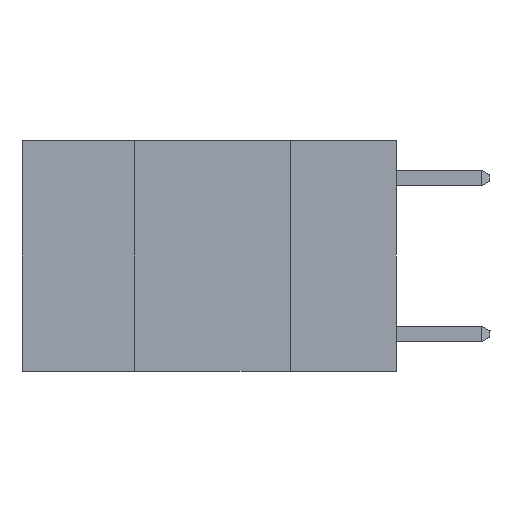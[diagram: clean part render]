
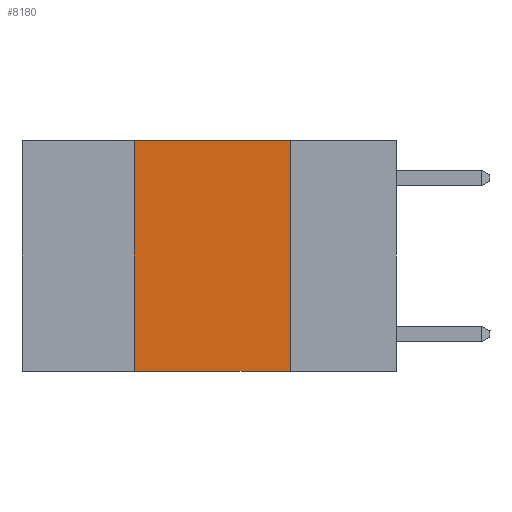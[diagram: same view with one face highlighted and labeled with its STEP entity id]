
A CAD part, left-side view. The second image highlights one B-rep face of the part: STEP entity #8180.
In plain terms, the highlighted planar face has unit normal (-1, 0, 0).
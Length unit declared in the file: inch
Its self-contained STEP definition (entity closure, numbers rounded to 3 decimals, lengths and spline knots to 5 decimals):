
#717 = CARTESIAN_POINT ( 'NONE',  ( 0., 0.42, 0. ) ) ;
#857 = LINE ( 'NONE', #12885, #6156 ) ;
#988 = CARTESIAN_POINT ( 'NONE',  ( 0., 0.6, -0.37 ) ) ;
#1146 = PLANE ( 'NONE',  #7755 ) ;
#1950 = LINE ( 'NONE', #988, #4448 ) ;
#2814 = CARTESIAN_POINT ( 'NONE',  ( 0., 0.17, 0. ) ) ;
#3198 = VERTEX_POINT ( 'NONE', #9468 ) ;
#3977 = EDGE_LOOP ( 'NONE', ( #6904, #7566, #7643, #7690 ) ) ;
#3981 = VERTEX_POINT ( 'NONE', #2814 ) ;
#4067 = CARTESIAN_POINT ( 'NONE',  ( 0., 0.6, 0. ) ) ;
#4317 = LINE ( 'NONE', #4067, #6766 ) ;
#4362 = DIRECTION ( 'NONE',  ( 0., 0., -1. ) ) ;
#4448 = VECTOR ( 'NONE', #9433, 39.37008 ) ;
#4833 = DIRECTION ( 'NONE',  ( 0., 0., -1. ) ) ;
#5678 = LINE ( 'NONE', #717, #8162 ) ;
#6156 = VECTOR ( 'NONE', #4833, 39.37008 ) ;
#6433 = VERTEX_POINT ( 'NONE', #10894 ) ;
#6766 = VECTOR ( 'NONE', #12214, 39.37008 ) ;
#6904 = ORIENTED_EDGE ( 'NONE', *, *, #11241, .F. ) ;
#7488 = CARTESIAN_POINT ( 'NONE',  ( 0., 0.6, 0. ) ) ;
#7541 = FACE_OUTER_BOUND ( 'NONE', #3977, .T. ) ;
#7566 = ORIENTED_EDGE ( 'NONE', *, *, #12040, .F. ) ;
#7643 = ORIENTED_EDGE ( 'NONE', *, *, #10610, .F. ) ;
#7690 = ORIENTED_EDGE ( 'NONE', *, *, #13126, .T. ) ;
#7755 = AXIS2_PLACEMENT_3D ( 'NONE', #7488, #10593, #4362 ) ;
#8162 = VECTOR ( 'NONE', #11092, 39.37008 ) ;
#8180 = ADVANCED_FACE ( 'NONE', ( #7541 ), #1146, .F. ) ;
#9433 = DIRECTION ( 'NONE',  ( 0., -1., 0. ) ) ;
#9468 = CARTESIAN_POINT ( 'NONE',  ( 0., 0.42, -0.37 ) ) ;
#9694 = CARTESIAN_POINT ( 'NONE',  ( 0., 0.17, -0.37 ) ) ;
#10593 = DIRECTION ( 'NONE',  ( 1., 0., 0. ) ) ;
#10610 = EDGE_CURVE ( 'NONE', #3198, #6433, #5678, .T. ) ;
#10894 = CARTESIAN_POINT ( 'NONE',  ( 0., 0.42, 0. ) ) ;
#11092 = DIRECTION ( 'NONE',  ( 0., 0., 1. ) ) ;
#11241 = EDGE_CURVE ( 'NONE', #3981, #12264, #857, .T. ) ;
#12040 = EDGE_CURVE ( 'NONE', #6433, #3981, #4317, .T. ) ;
#12214 = DIRECTION ( 'NONE',  ( 0., -1., 0. ) ) ;
#12264 = VERTEX_POINT ( 'NONE', #9694 ) ;
#12885 = CARTESIAN_POINT ( 'NONE',  ( 0., 0.17, 0. ) ) ;
#13126 = EDGE_CURVE ( 'NONE', #3198, #12264, #1950, .T. ) ;
